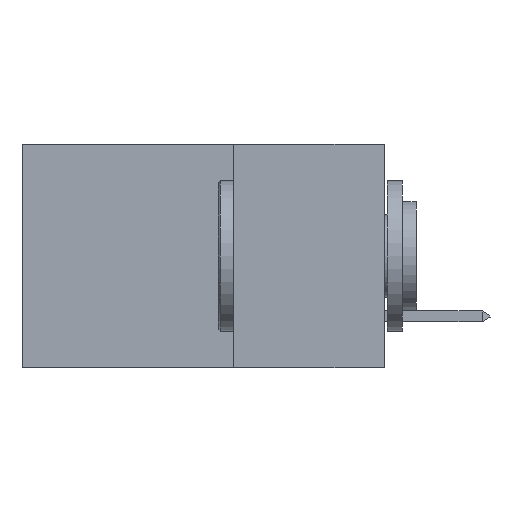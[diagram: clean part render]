
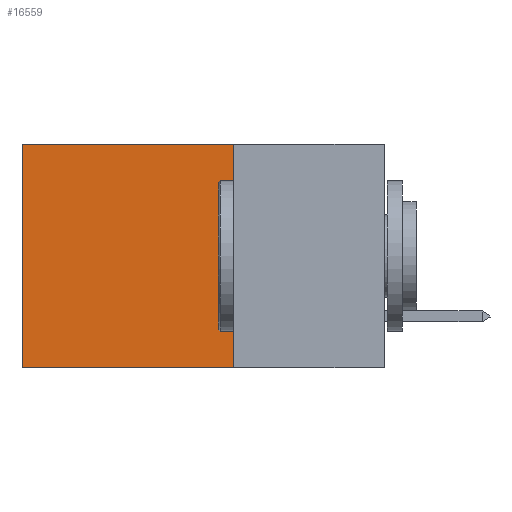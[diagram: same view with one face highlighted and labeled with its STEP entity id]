
A CAD part, left-side view. The second image highlights one B-rep face of the part: STEP entity #16559.
In plain terms, the highlighted planar face has unit normal (-1, 0, 0).
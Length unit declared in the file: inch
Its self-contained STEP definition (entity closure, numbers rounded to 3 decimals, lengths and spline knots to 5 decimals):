
#170 = EDGE_CURVE ( 'NONE', #3207, #4656, #8493, .T. ) ;
#316 = CARTESIAN_POINT ( 'NONE',  ( 0.2875, 0.25, -0.37 ) ) ;
#325 = AXIS2_PLACEMENT_3D ( 'NONE', #13001, #21989, #2275 ) ;
#1821 = VECTOR ( 'NONE', #18202, 39.37008 ) ;
#2275 = DIRECTION ( 'NONE',  ( 0., 0., -1. ) ) ;
#2395 = CARTESIAN_POINT ( 'NONE',  ( 0.2875, 0.25, 0. ) ) ;
#2400 = FACE_OUTER_BOUND ( 'NONE', #7542, .T. ) ;
#2451 = ORIENTED_EDGE ( 'NONE', *, *, #170, .T. ) ;
#2555 = LINE ( 'NONE', #18900, #3934 ) ;
#2957 = CARTESIAN_POINT ( 'NONE',  ( 0.2875, 0.6, 0. ) ) ;
#3207 = VERTEX_POINT ( 'NONE', #4111 ) ;
#3934 = VECTOR ( 'NONE', #22537, 39.37008 ) ;
#4111 = CARTESIAN_POINT ( 'NONE',  ( 0.2875, 0.25, 0. ) ) ;
#4656 = VERTEX_POINT ( 'NONE', #6870 ) ;
#5226 = VERTEX_POINT ( 'NONE', #11616 ) ;
#5353 = EDGE_CURVE ( 'NONE', #3207, #5226, #2555, .T. ) ;
#5583 = VECTOR ( 'NONE', #11962, 39.37008 ) ;
#6153 = DIRECTION ( 'NONE',  ( 0., 1., 0. ) ) ;
#6722 = ORIENTED_EDGE ( 'NONE', *, *, #7081, .T. ) ;
#6870 = CARTESIAN_POINT ( 'NONE',  ( 0.2875, 0.6, 0. ) ) ;
#7081 = EDGE_CURVE ( 'NONE', #4656, #17729, #22300, .T. ) ;
#7542 = EDGE_LOOP ( 'NONE', ( #6722, #22518, #21239, #2451 ) ) ;
#8493 = LINE ( 'NONE', #2395, #19326 ) ;
#8496 = CARTESIAN_POINT ( 'NONE',  ( 0.2875, 0.6, -0.37 ) ) ;
#11616 = CARTESIAN_POINT ( 'NONE',  ( 0.2875, 0.25, -0.37 ) ) ;
#11962 = DIRECTION ( 'NONE',  ( 0., 0., -1. ) ) ;
#13001 = CARTESIAN_POINT ( 'NONE',  ( 0.2875, 0.25, 0. ) ) ;
#16517 = EDGE_CURVE ( 'NONE', #5226, #17729, #16643, .T. ) ;
#16546 = PLANE ( 'NONE',  #325 ) ;
#16559 = ADVANCED_FACE ( 'NONE', ( #2400 ), #16546, .F. ) ;
#16643 = LINE ( 'NONE', #316, #1821 ) ;
#17729 = VERTEX_POINT ( 'NONE', #8496 ) ;
#18202 = DIRECTION ( 'NONE',  ( 0., 1., 0. ) ) ;
#18900 = CARTESIAN_POINT ( 'NONE',  ( 0.2875, 0.25, 0. ) ) ;
#19326 = VECTOR ( 'NONE', #6153, 39.37008 ) ;
#21239 = ORIENTED_EDGE ( 'NONE', *, *, #5353, .F. ) ;
#21989 = DIRECTION ( 'NONE',  ( 1., 0., 0. ) ) ;
#22300 = LINE ( 'NONE', #2957, #5583 ) ;
#22518 = ORIENTED_EDGE ( 'NONE', *, *, #16517, .F. ) ;
#22537 = DIRECTION ( 'NONE',  ( 0., 0., -1. ) ) ;
